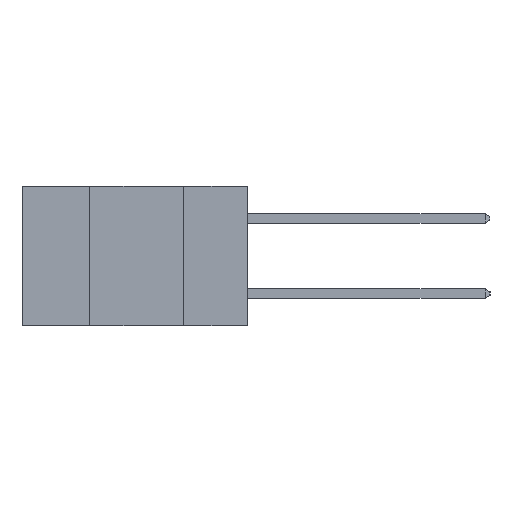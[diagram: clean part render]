
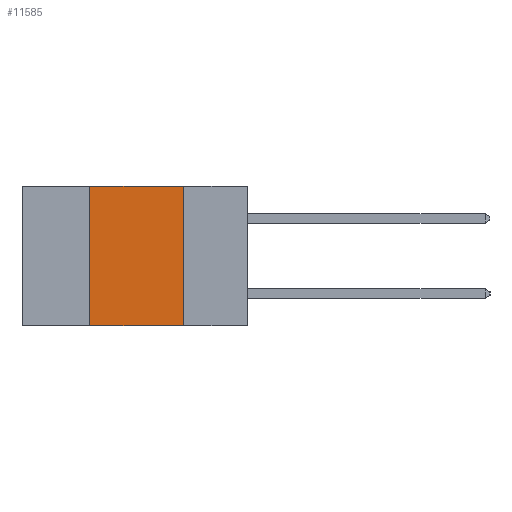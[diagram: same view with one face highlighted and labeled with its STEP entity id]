
A CAD part, left-side view. The second image highlights one B-rep face of the part: STEP entity #11585.
In plain terms, the highlighted planar face has unit normal (-1, 0, 0).
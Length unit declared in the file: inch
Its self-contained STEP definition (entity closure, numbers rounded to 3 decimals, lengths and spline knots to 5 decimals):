
#684 = DIRECTION ( 'NONE',  ( 0., 0., -1. ) ) ;
#1122 = EDGE_CURVE ( 'NONE', #13635, #9487, #7708, .T. ) ;
#1151 = ORIENTED_EDGE ( 'NONE', *, *, #1122, .T. ) ;
#2123 = FACE_OUTER_BOUND ( 'NONE', #11226, .T. ) ;
#2684 = VECTOR ( 'NONE', #5962, 39.37008 ) ;
#3081 = LINE ( 'NONE', #11069, #2684 ) ;
#3148 = ORIENTED_EDGE ( 'NONE', *, *, #14074, .F. ) ;
#3515 = LINE ( 'NONE', #8082, #9903 ) ;
#3680 = VECTOR ( 'NONE', #13999, 39.37008 ) ;
#3822 = CARTESIAN_POINT ( 'NONE',  ( 0., 0.6, 0. ) ) ;
#3864 = EDGE_CURVE ( 'NONE', #13635, #6487, #3081, .T. ) ;
#4613 = CARTESIAN_POINT ( 'NONE',  ( 0., 0.17, 0. ) ) ;
#4715 = VECTOR ( 'NONE', #9340, 39.37008 ) ;
#5715 = PLANE ( 'NONE',  #13839 ) ;
#5962 = DIRECTION ( 'NONE',  ( 0., 0., 1. ) ) ;
#6051 = CARTESIAN_POINT ( 'NONE',  ( 0., 0.42, 0. ) ) ;
#6487 = VERTEX_POINT ( 'NONE', #6051 ) ;
#6808 = DIRECTION ( 'NONE',  ( 0., 0., -1. ) ) ;
#7068 = LINE ( 'NONE', #3822, #3680 ) ;
#7708 = LINE ( 'NONE', #8971, #4715 ) ;
#8082 = CARTESIAN_POINT ( 'NONE',  ( 0., 0.17, -0.37 ) ) ;
#8274 = DIRECTION ( 'NONE',  ( 1., 0., 0. ) ) ;
#8971 = CARTESIAN_POINT ( 'NONE',  ( 0., 0.6, -0.37 ) ) ;
#9340 = DIRECTION ( 'NONE',  ( 0., -1., 0. ) ) ;
#9487 = VERTEX_POINT ( 'NONE', #14343 ) ;
#9506 = CARTESIAN_POINT ( 'NONE',  ( 0., 0.42, -0.37 ) ) ;
#9521 = ORIENTED_EDGE ( 'NONE', *, *, #11938, .F. ) ;
#9903 = VECTOR ( 'NONE', #6808, 39.37008 ) ;
#11069 = CARTESIAN_POINT ( 'NONE',  ( 0., 0.42, -0.37 ) ) ;
#11226 = EDGE_LOOP ( 'NONE', ( #3148, #9521, #11340, #1151 ) ) ;
#11340 = ORIENTED_EDGE ( 'NONE', *, *, #3864, .F. ) ;
#11585 = ADVANCED_FACE ( 'NONE', ( #2123 ), #5715, .F. ) ;
#11938 = EDGE_CURVE ( 'NONE', #6487, #14271, #7068, .T. ) ;
#13635 = VERTEX_POINT ( 'NONE', #9506 ) ;
#13839 = AXIS2_PLACEMENT_3D ( 'NONE', #15876, #8274, #684 ) ;
#13999 = DIRECTION ( 'NONE',  ( 0., -1., 0. ) ) ;
#14074 = EDGE_CURVE ( 'NONE', #14271, #9487, #3515, .T. ) ;
#14271 = VERTEX_POINT ( 'NONE', #4613 ) ;
#14343 = CARTESIAN_POINT ( 'NONE',  ( 0., 0.17, -0.37 ) ) ;
#15876 = CARTESIAN_POINT ( 'NONE',  ( 0., 0.6, 0. ) ) ;
